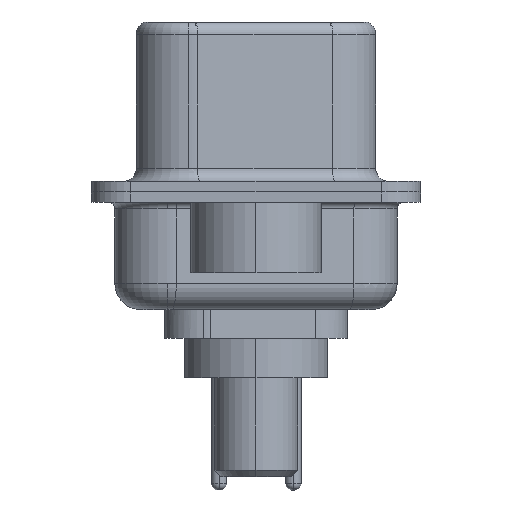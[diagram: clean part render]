
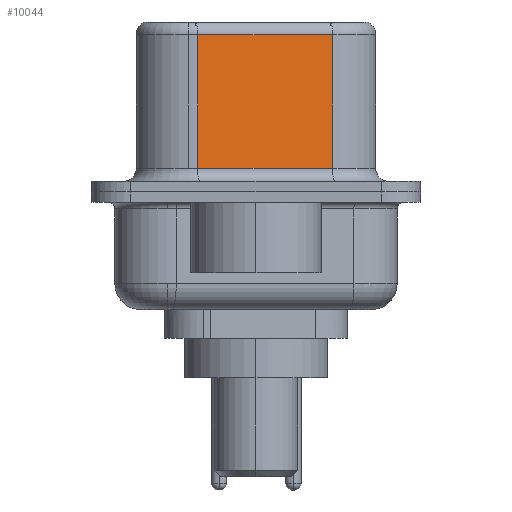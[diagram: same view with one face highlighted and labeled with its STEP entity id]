
A CAD part, left-side view. The second image highlights one B-rep face of the part: STEP entity #10044.
In plain terms, the highlighted planar face has unit normal (-0.985, -0.174, 0).
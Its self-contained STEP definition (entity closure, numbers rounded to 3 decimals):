
#1058 = VECTOR ( 'NONE', #21719, 1000. ) ;
#1484 = AXIS2_PLACEMENT_3D ( 'NONE', #14076, #7401, #19212 ) ;
#2071 = CARTESIAN_POINT ( 'NONE',  ( 4.58, -2.927, 0.9 ) ) ;
#3477 = LINE ( 'NONE', #16382, #3999 ) ;
#3999 = VECTOR ( 'NONE', #19742, 1000. ) ;
#5136 = VECTOR ( 'NONE', #11855, 1000. ) ;
#7108 = ORIENTED_EDGE ( 'NONE', *, *, #8664, .T. ) ;
#7218 = ORIENTED_EDGE ( 'NONE', *, *, #17318, .T. ) ;
#7401 = DIRECTION ( 'NONE',  ( 0.985, 0.174, 0. ) ) ;
#7861 = VERTEX_POINT ( 'NONE', #19713 ) ;
#8664 = EDGE_CURVE ( 'NONE', #9874, #21928, #3477, .T. ) ;
#9859 = CARTESIAN_POINT ( 'NONE',  ( 4.58, -2.927, 6.02 ) ) ;
#9874 = VERTEX_POINT ( 'NONE', #17059 ) ;
#10044 = ADVANCED_FACE ( 'NONE', ( #21150 ), #17493, .F. ) ;
#10058 = LINE ( 'NONE', #9859, #1058 ) ;
#11588 = VERTEX_POINT ( 'NONE', #14027 ) ;
#11855 = DIRECTION ( 'NONE',  ( 0., 0., -1. ) ) ;
#12586 = EDGE_CURVE ( 'NONE', #11588, #21928, #18652, .T. ) ;
#13960 = ORIENTED_EDGE ( 'NONE', *, *, #12586, .F. ) ;
#14027 = CARTESIAN_POINT ( 'NONE',  ( 4.58, -2.927, 6.02 ) ) ;
#14076 = CARTESIAN_POINT ( 'NONE',  ( 4.58, -2.927, 6.52 ) ) ;
#15084 = ORIENTED_EDGE ( 'NONE', *, *, #21325, .T. ) ;
#15186 = CARTESIAN_POINT ( 'NONE',  ( 4.58, -2.927, 6.52 ) ) ;
#16382 = CARTESIAN_POINT ( 'NONE',  ( 4.58, -2.927, 0.9 ) ) ;
#17059 = CARTESIAN_POINT ( 'NONE',  ( 3.67, 2.233, 0.9 ) ) ;
#17318 = EDGE_CURVE ( 'NONE', #7861, #9874, #17519, .T. ) ;
#17493 = PLANE ( 'NONE',  #1484 ) ;
#17519 = LINE ( 'NONE', #20308, #5136 ) ;
#18652 = LINE ( 'NONE', #15186, #19177 ) ;
#18708 = EDGE_LOOP ( 'NONE', ( #13960, #15084, #7218, #7108 ) ) ;
#19177 = VECTOR ( 'NONE', #20251, 1000. ) ;
#19212 = DIRECTION ( 'NONE',  ( -0.174, 0.985, 0. ) ) ;
#19713 = CARTESIAN_POINT ( 'NONE',  ( 3.67, 2.233, 6.02 ) ) ;
#19742 = DIRECTION ( 'NONE',  ( 0.174, -0.985, 0. ) ) ;
#20251 = DIRECTION ( 'NONE',  ( 0., 0., -1. ) ) ;
#20308 = CARTESIAN_POINT ( 'NONE',  ( 3.67, 2.233, 6.52 ) ) ;
#21150 = FACE_OUTER_BOUND ( 'NONE', #18708, .T. ) ;
#21325 = EDGE_CURVE ( 'NONE', #11588, #7861, #10058, .T. ) ;
#21719 = DIRECTION ( 'NONE',  ( -0.174, 0.985, 0. ) ) ;
#21928 = VERTEX_POINT ( 'NONE', #2071 ) ;
